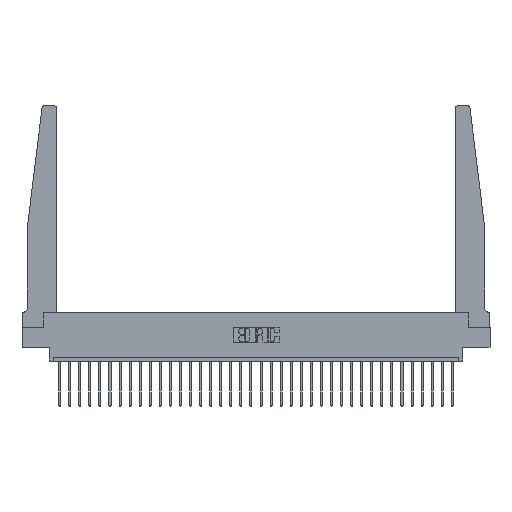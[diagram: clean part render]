
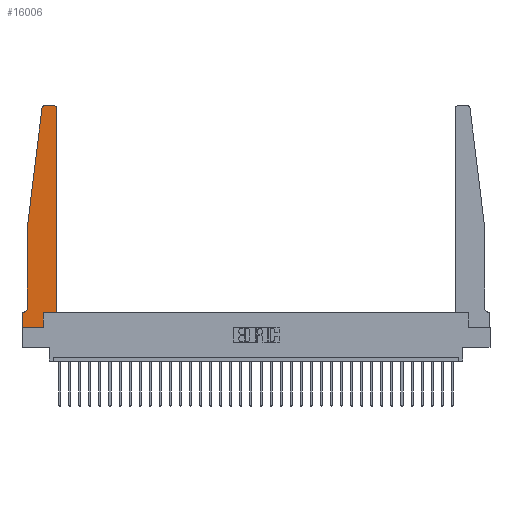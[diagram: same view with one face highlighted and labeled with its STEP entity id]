
A CAD part, top view. The second image highlights one B-rep face of the part: STEP entity #16006.
In plain terms, the highlighted planar face has unit normal (0, 0, 1).
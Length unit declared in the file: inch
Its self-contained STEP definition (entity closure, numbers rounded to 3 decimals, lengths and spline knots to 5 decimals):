
#501 = EDGE_CURVE ( 'NONE', #8927, #3555, #13778, .T. ) ;
#551 = AXIS2_PLACEMENT_3D ( 'NONE', #610, #19210, #16600 ) ;
#610 = CARTESIAN_POINT ( 'NONE',  ( 0., 0.1875, 0.37 ) ) ;
#1145 = CARTESIAN_POINT ( 'NONE',  ( 0.27653, 2.75, 0.37 ) ) ;
#1234 = EDGE_CURVE ( 'NONE', #6860, #1815, #11847, .T. ) ;
#1332 = AXIS2_PLACEMENT_3D ( 'NONE', #29161, #29457, #27466 ) ;
#1438 = VECTOR ( 'NONE', #28658, 39.37008 ) ;
#1462 = CARTESIAN_POINT ( 'NONE',  ( 0., 0., 0.37 ) ) ;
#1638 = CARTESIAN_POINT ( 'NONE',  ( 0.2605, 0.18, 0.37 ) ) ;
#1815 = VERTEX_POINT ( 'NONE', #19890 ) ;
#2035 = EDGE_CURVE ( 'NONE', #12993, #21169, #23608, .T. ) ;
#2076 = CARTESIAN_POINT ( 'NONE',  ( 0.2605, 0.18, 0.37 ) ) ;
#2107 = LINE ( 'NONE', #23353, #11861 ) ;
#2178 = VERTEX_POINT ( 'NONE', #14816 ) ;
#3555 = VERTEX_POINT ( 'NONE', #23264 ) ;
#3750 = DIRECTION ( 'NONE',  ( -1., 0., 0. ) ) ;
#3783 = VECTOR ( 'NONE', #25308, 39.37008 ) ;
#3901 = ORIENTED_EDGE ( 'NONE', *, *, #1234, .T. ) ;
#5003 = EDGE_CURVE ( 'NONE', #26944, #6986, #2107, .T. ) ;
#5214 = VECTOR ( 'NONE', #21048, 39.37008 ) ;
#5580 = LINE ( 'NONE', #14819, #14165 ) ;
#6613 = ORIENTED_EDGE ( 'NONE', *, *, #25850, .T. ) ;
#6666 = DIRECTION ( 'NONE',  ( -1., 0., 0. ) ) ;
#6690 = AXIS2_PLACEMENT_3D ( 'NONE', #22566, #15621, #13466 ) ;
#6860 = VERTEX_POINT ( 'NONE', #12672 ) ;
#6877 = DIRECTION ( 'NONE',  ( 0., 1., 0. ) ) ;
#6986 = VERTEX_POINT ( 'NONE', #12964 ) ;
#7185 = CIRCLE ( 'NONE', #6690, 0.03 ) ;
#7225 = VERTEX_POINT ( 'NONE', #16492 ) ;
#7235 = VECTOR ( 'NONE', #11759, 39.37008 ) ;
#7296 = EDGE_CURVE ( 'NONE', #6986, #12993, #10094, .T. ) ;
#7425 = DIRECTION ( 'NONE',  ( 1., 0., 0. ) ) ;
#8637 = VECTOR ( 'NONE', #6666, 39.37008 ) ;
#8927 = VERTEX_POINT ( 'NONE', #1462 ) ;
#10094 = CIRCLE ( 'NONE', #10593, 0.03 ) ;
#10593 = AXIS2_PLACEMENT_3D ( 'NONE', #19110, #28537, #7425 ) ;
#11272 = ORIENTED_EDGE ( 'NONE', *, *, #11873, .T. ) ;
#11652 = CARTESIAN_POINT ( 'NONE',  ( 0.065, 1.25, 0.37 ) ) ;
#11759 = DIRECTION ( 'NONE',  ( 1., 0., 0. ) ) ;
#11847 = LINE ( 'NONE', #19226, #1438 ) ;
#11861 = VECTOR ( 'NONE', #6877, 39.37008 ) ;
#11873 = EDGE_CURVE ( 'NONE', #21169, #2178, #7185, .T. ) ;
#11977 = VERTEX_POINT ( 'NONE', #2076 ) ;
#12306 = EDGE_CURVE ( 'NONE', #1815, #14980, #19019, .T. ) ;
#12457 = EDGE_CURVE ( 'NONE', #11977, #26944, #27770, .T. ) ;
#12672 = CARTESIAN_POINT ( 'NONE',  ( 0.065, 1.25, 0.37 ) ) ;
#12839 = CARTESIAN_POINT ( 'NONE',  ( 0.015, 0.1875, 0.37 ) ) ;
#12866 = DIRECTION ( 'NONE',  ( 0., 1., 0. ) ) ;
#12877 = EDGE_CURVE ( 'NONE', #7225, #8927, #5580, .T. ) ;
#12964 = CARTESIAN_POINT ( 'NONE',  ( 0.425, 2.72, 0.37 ) ) ;
#12993 = VERTEX_POINT ( 'NONE', #25858 ) ;
#13466 = DIRECTION ( 'NONE',  ( 1., 0., 0. ) ) ;
#13718 = EDGE_CURVE ( 'NONE', #14980, #7225, #15448, .T. ) ;
#13778 = LINE ( 'NONE', #30413, #7235 ) ;
#14165 = VECTOR ( 'NONE', #24229, 39.37008 ) ;
#14816 = CARTESIAN_POINT ( 'NONE',  ( 0.24675, 2.72367, 0.37 ) ) ;
#14819 = CARTESIAN_POINT ( 'NONE',  ( 0., 0., 0.37 ) ) ;
#14980 = VERTEX_POINT ( 'NONE', #12839 ) ;
#15448 = LINE ( 'NONE', #17911, #26524 ) ;
#15621 = DIRECTION ( 'NONE',  ( 0., 0., 1. ) ) ;
#16006 = ADVANCED_FACE ( 'NONE', ( #23859 ), #24015, .T. ) ;
#16229 = VECTOR ( 'NONE', #12866, 39.37008 ) ;
#16481 = ORIENTED_EDGE ( 'NONE', *, *, #12877, .T. ) ;
#16492 = CARTESIAN_POINT ( 'NONE',  ( 0., 0.1875, 0.37 ) ) ;
#16600 = DIRECTION ( 'NONE',  ( 1., 0., 0. ) ) ;
#17197 = ORIENTED_EDGE ( 'NONE', *, *, #12457, .T. ) ;
#17316 = ORIENTED_EDGE ( 'NONE', *, *, #501, .T. ) ;
#17815 = ORIENTED_EDGE ( 'NONE', *, *, #13718, .T. ) ;
#17911 = CARTESIAN_POINT ( 'NONE',  ( 0.065, 0.1875, 0.37 ) ) ;
#17944 = LINE ( 'NONE', #1638, #16229 ) ;
#18301 = ORIENTED_EDGE ( 'NONE', *, *, #5003, .T. ) ;
#18808 = EDGE_CURVE ( 'NONE', #2178, #6860, #18889, .T. ) ;
#18889 = LINE ( 'NONE', #11652, #5214 ) ;
#19019 = CIRCLE ( 'NONE', #1332, 0.05 ) ;
#19110 = CARTESIAN_POINT ( 'NONE',  ( 0.395, 2.72, 0.37 ) ) ;
#19210 = DIRECTION ( 'NONE',  ( 0., 0., 1. ) ) ;
#19226 = CARTESIAN_POINT ( 'NONE',  ( 0.065, 1.25, 0.37 ) ) ;
#19890 = CARTESIAN_POINT ( 'NONE',  ( 0.065, 0.2375, 0.37 ) ) ;
#20977 = CARTESIAN_POINT ( 'NONE',  ( 0.25, 2.75, 0.37 ) ) ;
#21048 = DIRECTION ( 'NONE',  ( -0.122, -0.992, 0. ) ) ;
#21127 = CARTESIAN_POINT ( 'NONE',  ( 0.425, 0.18, 0.37 ) ) ;
#21169 = VERTEX_POINT ( 'NONE', #1145 ) ;
#21410 = CARTESIAN_POINT ( 'NONE',  ( 0.425, 0.18, 0.37 ) ) ;
#22566 = CARTESIAN_POINT ( 'NONE',  ( 0.27653, 2.72, 0.37 ) ) ;
#23264 = CARTESIAN_POINT ( 'NONE',  ( 0.2605, 0., 0.37 ) ) ;
#23353 = CARTESIAN_POINT ( 'NONE',  ( 0.425, 0.18, 0.37 ) ) ;
#23608 = LINE ( 'NONE', #20977, #8637 ) ;
#23859 = FACE_OUTER_BOUND ( 'NONE', #30063, .T. ) ;
#24015 = PLANE ( 'NONE',  #551 ) ;
#24229 = DIRECTION ( 'NONE',  ( 0., -1., 0. ) ) ;
#25308 = DIRECTION ( 'NONE',  ( 1., 0., 0. ) ) ;
#25846 = ORIENTED_EDGE ( 'NONE', *, *, #7296, .T. ) ;
#25850 = EDGE_CURVE ( 'NONE', #3555, #11977, #17944, .T. ) ;
#25858 = CARTESIAN_POINT ( 'NONE',  ( 0.395, 2.75, 0.37 ) ) ;
#26524 = VECTOR ( 'NONE', #3750, 39.37008 ) ;
#26944 = VERTEX_POINT ( 'NONE', #21410 ) ;
#27043 = ORIENTED_EDGE ( 'NONE', *, *, #18808, .T. ) ;
#27466 = DIRECTION ( 'NONE',  ( -1., 0., 0. ) ) ;
#27770 = LINE ( 'NONE', #21127, #3783 ) ;
#28537 = DIRECTION ( 'NONE',  ( 0., 0., 1. ) ) ;
#28658 = DIRECTION ( 'NONE',  ( 0., -1., 0. ) ) ;
#28757 = ORIENTED_EDGE ( 'NONE', *, *, #12306, .T. ) ;
#29161 = CARTESIAN_POINT ( 'NONE',  ( 0.015, 0.2375, 0.37 ) ) ;
#29409 = ORIENTED_EDGE ( 'NONE', *, *, #2035, .T. ) ;
#29457 = DIRECTION ( 'NONE',  ( 0., 0., -1. ) ) ;
#30063 = EDGE_LOOP ( 'NONE', ( #29409, #11272, #27043, #3901, #28757, #17815, #16481, #17316, #6613, #17197, #18301, #25846 ) ) ;
#30413 = CARTESIAN_POINT ( 'NONE',  ( 0., 0., 0.37 ) ) ;
